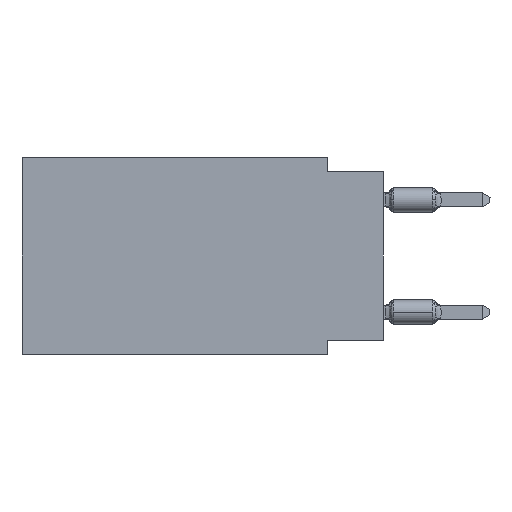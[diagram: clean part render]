
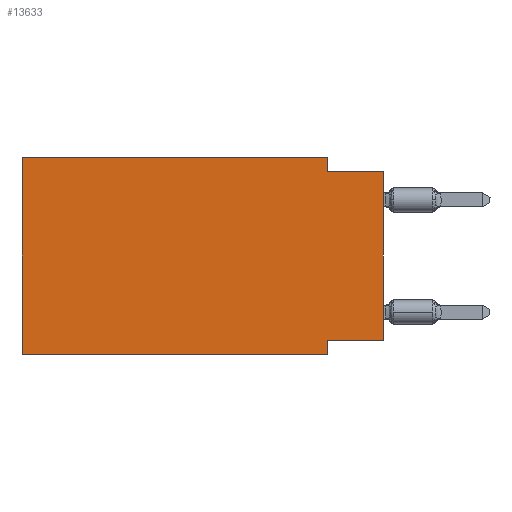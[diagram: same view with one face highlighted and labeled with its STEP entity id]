
A CAD part, left-side view. The second image highlights one B-rep face of the part: STEP entity #13633.
In plain terms, the highlighted planar face has unit normal (-1, 0, 0).
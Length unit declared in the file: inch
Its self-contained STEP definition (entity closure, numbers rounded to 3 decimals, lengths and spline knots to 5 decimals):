
#295 = VERTEX_POINT ( 'NONE', #5790 ) ;
#541 = ORIENTED_EDGE ( 'NONE', *, *, #35578, .T. ) ;
#3115 = PLANE ( 'NONE',  #31638 ) ;
#3338 = EDGE_LOOP ( 'NONE', ( #541, #34910, #5532, #9708, #39522, #29512, #25362, #45522 ) ) ;
#4798 = DIRECTION ( 'NONE',  ( 0., 0., -1. ) ) ;
#5532 = ORIENTED_EDGE ( 'NONE', *, *, #33132, .F. ) ;
#5790 = CARTESIAN_POINT ( 'NONE',  ( 0., 0.645, -0.35 ) ) ;
#6086 = LINE ( 'NONE', #30066, #26634 ) ;
#6930 = LINE ( 'NONE', #23448, #21755 ) ;
#7985 = CARTESIAN_POINT ( 'NONE',  ( 0., 0., -0.325 ) ) ;
#8058 = LINE ( 'NONE', #36202, #43339 ) ;
#8192 = VECTOR ( 'NONE', #44487, 39.37008 ) ;
#8492 = DIRECTION ( 'NONE',  ( 0., -1., 0. ) ) ;
#8979 = VERTEX_POINT ( 'NONE', #17318 ) ;
#9708 = ORIENTED_EDGE ( 'NONE', *, *, #42809, .F. ) ;
#9816 = DIRECTION ( 'NONE',  ( 0., -1., 0. ) ) ;
#10183 = VERTEX_POINT ( 'NONE', #30308 ) ;
#12757 = LINE ( 'NONE', #20555, #8192 ) ;
#13304 = FACE_OUTER_BOUND ( 'NONE', #3338, .T. ) ;
#13633 = ADVANCED_FACE ( 'NONE', ( #13304 ), #3115, .F. ) ;
#13690 = CARTESIAN_POINT ( 'NONE',  ( 0., 0.1, -0.325 ) ) ;
#14909 = EDGE_CURVE ( 'NONE', #20693, #22171, #8058, .T. ) ;
#15627 = DIRECTION ( 'NONE',  ( 0., 1., 0. ) ) ;
#16144 = LINE ( 'NONE', #30171, #20138 ) ;
#17318 = CARTESIAN_POINT ( 'NONE',  ( 0., 0.645, 0. ) ) ;
#18533 = DIRECTION ( 'NONE',  ( 0., 0., -1. ) ) ;
#18595 = LINE ( 'NONE', #7985, #42603 ) ;
#20138 = VECTOR ( 'NONE', #8492, 39.37008 ) ;
#20555 = CARTESIAN_POINT ( 'NONE',  ( 0., 0., 0. ) ) ;
#20693 = VERTEX_POINT ( 'NONE', #13690 ) ;
#21755 = VECTOR ( 'NONE', #9816, 39.37008 ) ;
#22171 = VERTEX_POINT ( 'NONE', #25165 ) ;
#22685 = DIRECTION ( 'NONE',  ( 0., -1., 0. ) ) ;
#23448 = CARTESIAN_POINT ( 'NONE',  ( 0., 0.645, 0. ) ) ;
#24351 = CARTESIAN_POINT ( 'NONE',  ( 0., 0.645, 0. ) ) ;
#24391 = VERTEX_POINT ( 'NONE', #33626 ) ;
#24693 = EDGE_CURVE ( 'NONE', #24391, #20693, #18595, .T. ) ;
#25165 = CARTESIAN_POINT ( 'NONE',  ( 0., 0.1, -0.35 ) ) ;
#25362 = ORIENTED_EDGE ( 'NONE', *, *, #14909, .F. ) ;
#26148 = CARTESIAN_POINT ( 'NONE',  ( 0., 0., -0.025 ) ) ;
#26634 = VECTOR ( 'NONE', #41075, 39.37008 ) ;
#28241 = DIRECTION ( 'NONE',  ( 1., 0., 0. ) ) ;
#29104 = CARTESIAN_POINT ( 'NONE',  ( 0., 0.1, 0. ) ) ;
#29176 = CARTESIAN_POINT ( 'NONE',  ( 0., 0.1, -0.025 ) ) ;
#29512 = ORIENTED_EDGE ( 'NONE', *, *, #40335, .T. ) ;
#29873 = VECTOR ( 'NONE', #18533, 39.37008 ) ;
#30066 = CARTESIAN_POINT ( 'NONE',  ( 0., 0.645, 0. ) ) ;
#30171 = CARTESIAN_POINT ( 'NONE',  ( 0., 0.645, -0.35 ) ) ;
#30308 = CARTESIAN_POINT ( 'NONE',  ( 0., 0., -0.025 ) ) ;
#30334 = VERTEX_POINT ( 'NONE', #29176 ) ;
#30927 = EDGE_CURVE ( 'NONE', #30334, #10183, #43602, .T. ) ;
#31638 = AXIS2_PLACEMENT_3D ( 'NONE', #24351, #28241, #38828 ) ;
#32359 = CARTESIAN_POINT ( 'NONE',  ( 0., 0.1, 0. ) ) ;
#33132 = EDGE_CURVE ( 'NONE', #35492, #30334, #42444, .T. ) ;
#33626 = CARTESIAN_POINT ( 'NONE',  ( 0., 0., -0.325 ) ) ;
#34910 = ORIENTED_EDGE ( 'NONE', *, *, #30927, .F. ) ;
#35492 = VERTEX_POINT ( 'NONE', #29104 ) ;
#35578 = EDGE_CURVE ( 'NONE', #24391, #10183, #12757, .T. ) ;
#36202 = CARTESIAN_POINT ( 'NONE',  ( 0., 0.1, -0.35 ) ) ;
#38035 = EDGE_CURVE ( 'NONE', #295, #8979, #6086, .T. ) ;
#38828 = DIRECTION ( 'NONE',  ( 0., 0., -1. ) ) ;
#39522 = ORIENTED_EDGE ( 'NONE', *, *, #38035, .F. ) ;
#40335 = EDGE_CURVE ( 'NONE', #295, #22171, #16144, .T. ) ;
#41075 = DIRECTION ( 'NONE',  ( 0., 0., 1. ) ) ;
#42444 = LINE ( 'NONE', #32359, #29873 ) ;
#42603 = VECTOR ( 'NONE', #15627, 39.37008 ) ;
#42809 = EDGE_CURVE ( 'NONE', #8979, #35492, #6930, .T. ) ;
#43339 = VECTOR ( 'NONE', #4798, 39.37008 ) ;
#43602 = LINE ( 'NONE', #26148, #45506 ) ;
#44487 = DIRECTION ( 'NONE',  ( 0., 0., 1. ) ) ;
#45506 = VECTOR ( 'NONE', #22685, 39.37008 ) ;
#45522 = ORIENTED_EDGE ( 'NONE', *, *, #24693, .F. ) ;
